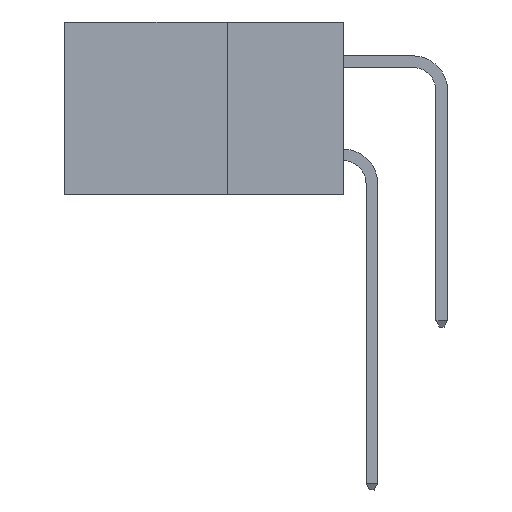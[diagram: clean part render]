
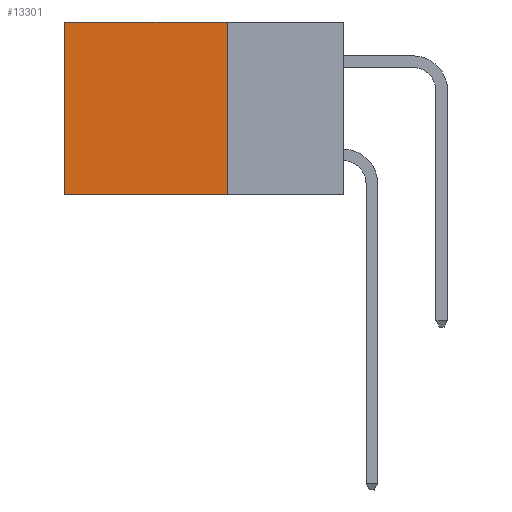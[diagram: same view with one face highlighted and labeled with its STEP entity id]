
A CAD part, left-side view. The second image highlights one B-rep face of the part: STEP entity #13301.
In plain terms, the highlighted planar face has unit normal (-1, 0, 0).
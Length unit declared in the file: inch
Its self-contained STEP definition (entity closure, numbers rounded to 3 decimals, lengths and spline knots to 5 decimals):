
#649 = ORIENTED_EDGE ( 'NONE', *, *, #1021, .F. ) ;
#1021 = EDGE_CURVE ( 'NONE', #11860, #11078, #13791, .T. ) ;
#1264 = DIRECTION ( 'NONE',  ( 0., 0., -1. ) ) ;
#1363 = ORIENTED_EDGE ( 'NONE', *, *, #18398, .T. ) ;
#1459 = VECTOR ( 'NONE', #13930, 39.37008 ) ;
#1989 = CARTESIAN_POINT ( 'NONE',  ( 0.298, 0.6, -0.37 ) ) ;
#2146 = CARTESIAN_POINT ( 'NONE',  ( 0.298, 0.6, 0. ) ) ;
#3903 = AXIS2_PLACEMENT_3D ( 'NONE', #8839, #16651, #11745 ) ;
#6178 = EDGE_CURVE ( 'NONE', #11860, #17546, #18518, .T. ) ;
#6309 = VECTOR ( 'NONE', #1264, 39.37008 ) ;
#6355 = CARTESIAN_POINT ( 'NONE',  ( 0.298, 0.25, -0.37 ) ) ;
#7451 = VECTOR ( 'NONE', #15815, 39.37008 ) ;
#8839 = CARTESIAN_POINT ( 'NONE',  ( 0.298, 0.25, 0. ) ) ;
#9141 = CARTESIAN_POINT ( 'NONE',  ( 0.298, 0.25, 0. ) ) ;
#9594 = LINE ( 'NONE', #6355, #7451 ) ;
#10557 = CARTESIAN_POINT ( 'NONE',  ( 0.298, 0.6, 0. ) ) ;
#11078 = VERTEX_POINT ( 'NONE', #17881 ) ;
#11306 = VERTEX_POINT ( 'NONE', #1989 ) ;
#11745 = DIRECTION ( 'NONE',  ( 0., 0., -1. ) ) ;
#11860 = VERTEX_POINT ( 'NONE', #18035 ) ;
#12150 = ORIENTED_EDGE ( 'NONE', *, *, #6178, .T. ) ;
#12293 = DIRECTION ( 'NONE',  ( 0., 1., 0. ) ) ;
#12397 = CARTESIAN_POINT ( 'NONE',  ( 0.298, 0.25, 0. ) ) ;
#13301 = ADVANCED_FACE ( 'NONE', ( #19593 ), #13347, .F. ) ;
#13347 = PLANE ( 'NONE',  #3903 ) ;
#13791 = LINE ( 'NONE', #12397, #1459 ) ;
#13930 = DIRECTION ( 'NONE',  ( 0., 0., -1. ) ) ;
#14760 = ORIENTED_EDGE ( 'NONE', *, *, #14976, .F. ) ;
#14976 = EDGE_CURVE ( 'NONE', #11078, #11306, #9594, .T. ) ;
#15815 = DIRECTION ( 'NONE',  ( 0., 1., 0. ) ) ;
#15891 = EDGE_LOOP ( 'NONE', ( #1363, #14760, #649, #12150 ) ) ;
#16651 = DIRECTION ( 'NONE',  ( 1., 0., 0. ) ) ;
#17537 = VECTOR ( 'NONE', #12293, 39.37008 ) ;
#17546 = VERTEX_POINT ( 'NONE', #2146 ) ;
#17881 = CARTESIAN_POINT ( 'NONE',  ( 0.298, 0.25, -0.37 ) ) ;
#18035 = CARTESIAN_POINT ( 'NONE',  ( 0.298, 0.25, 0. ) ) ;
#18398 = EDGE_CURVE ( 'NONE', #17546, #11306, #18424, .T. ) ;
#18424 = LINE ( 'NONE', #10557, #6309 ) ;
#18518 = LINE ( 'NONE', #9141, #17537 ) ;
#19593 = FACE_OUTER_BOUND ( 'NONE', #15891, .T. ) ;
